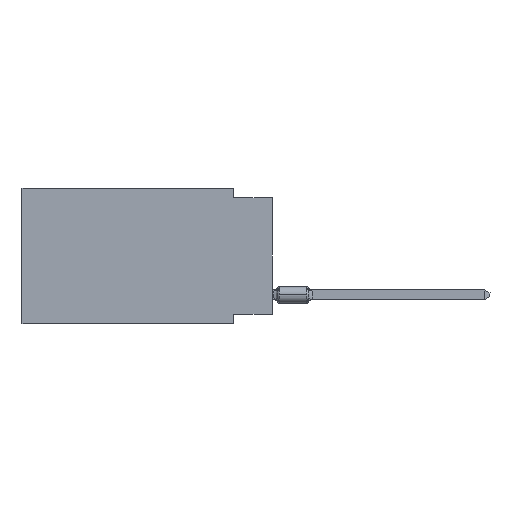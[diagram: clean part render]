
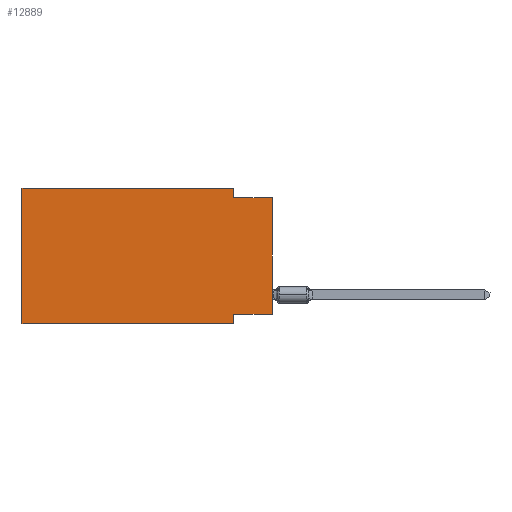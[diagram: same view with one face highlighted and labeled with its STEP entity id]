
A CAD part, left-side view. The second image highlights one B-rep face of the part: STEP entity #12889.
In plain terms, the highlighted planar face has unit normal (-1, 0, 0).
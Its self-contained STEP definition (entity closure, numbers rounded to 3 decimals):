
#615 = LINE ( 'NONE', #16042, #12600 ) ;
#970 = EDGE_CURVE ( 'NONE', #9840, #2239, #18600, .T. ) ;
#1143 = EDGE_CURVE ( 'NONE', #9840, #15726, #25029, .T. ) ;
#1150 = DIRECTION ( 'NONE',  ( 0., 0., -1. ) ) ;
#1346 = CARTESIAN_POINT ( 'NONE',  ( 0., 0., 0. ) ) ;
#1924 = CARTESIAN_POINT ( 'NONE',  ( 0., 16.383, -8.89 ) ) ;
#1976 = DIRECTION ( 'NONE',  ( 0., -1., 0. ) ) ;
#2064 = ORIENTED_EDGE ( 'NONE', *, *, #970, .F. ) ;
#2103 = LINE ( 'NONE', #22062, #3014 ) ;
#2239 = VERTEX_POINT ( 'NONE', #5810 ) ;
#2859 = VERTEX_POINT ( 'NONE', #17123 ) ;
#3014 = VECTOR ( 'NONE', #1976, 1000. ) ;
#3246 = ORIENTED_EDGE ( 'NONE', *, *, #18876, .F. ) ;
#3462 = EDGE_LOOP ( 'NONE', ( #14455, #17822, #12158, #16643, #3246, #7448, #14622, #2064 ) ) ;
#3702 = LINE ( 'NONE', #7567, #4175 ) ;
#4145 = FACE_OUTER_BOUND ( 'NONE', #3462, .T. ) ;
#4175 = VECTOR ( 'NONE', #11543, 1000. ) ;
#4711 = EDGE_CURVE ( 'NONE', #2239, #5932, #615, .T. ) ;
#4917 = EDGE_CURVE ( 'NONE', #11958, #22137, #24407, .T. ) ;
#5617 = CARTESIAN_POINT ( 'NONE',  ( 0., 16.383, 0. ) ) ;
#5810 = CARTESIAN_POINT ( 'NONE',  ( 0., 2.54, -8.255 ) ) ;
#5932 = VERTEX_POINT ( 'NONE', #16215 ) ;
#7036 = DIRECTION ( 'NONE',  ( 0., 0., -1. ) ) ;
#7448 = ORIENTED_EDGE ( 'NONE', *, *, #10541, .T. ) ;
#7567 = CARTESIAN_POINT ( 'NONE',  ( 0., 16.383, 0. ) ) ;
#8411 = VECTOR ( 'NONE', #8682, 1000. ) ;
#8682 = DIRECTION ( 'NONE',  ( 0., -1., 0. ) ) ;
#8826 = CARTESIAN_POINT ( 'NONE',  ( 0., 0., -8.255 ) ) ;
#9204 = DIRECTION ( 'NONE',  ( 0., 0., 1. ) ) ;
#9279 = DIRECTION ( 'NONE',  ( 0., -1., 0. ) ) ;
#9840 = VERTEX_POINT ( 'NONE', #21013 ) ;
#10541 = EDGE_CURVE ( 'NONE', #2859, #5932, #15173, .T. ) ;
#10889 = VECTOR ( 'NONE', #16668, 1000. ) ;
#11504 = EDGE_CURVE ( 'NONE', #22137, #15726, #2103, .T. ) ;
#11543 = DIRECTION ( 'NONE',  ( 0., 0., 1. ) ) ;
#11562 = CARTESIAN_POINT ( 'NONE',  ( 0., 0., -0.635 ) ) ;
#11958 = VERTEX_POINT ( 'NONE', #14538 ) ;
#12058 = CARTESIAN_POINT ( 'NONE',  ( 0., 2.54, -0.635 ) ) ;
#12158 = ORIENTED_EDGE ( 'NONE', *, *, #4917, .F. ) ;
#12600 = VECTOR ( 'NONE', #19667, 1000. ) ;
#12889 = ADVANCED_FACE ( 'NONE', ( #4145 ), #19583, .F. ) ;
#14253 = VECTOR ( 'NONE', #7036, 1000. ) ;
#14455 = ORIENTED_EDGE ( 'NONE', *, *, #1143, .T. ) ;
#14538 = CARTESIAN_POINT ( 'NONE',  ( 0., 2.54, 0. ) ) ;
#14582 = CARTESIAN_POINT ( 'NONE',  ( 0., 16.383, 0. ) ) ;
#14622 = ORIENTED_EDGE ( 'NONE', *, *, #4711, .F. ) ;
#15173 = LINE ( 'NONE', #1924, #21056 ) ;
#15726 = VERTEX_POINT ( 'NONE', #11562 ) ;
#16042 = CARTESIAN_POINT ( 'NONE',  ( 0., 2.54, -8.89 ) ) ;
#16215 = CARTESIAN_POINT ( 'NONE',  ( 0., 2.54, -8.89 ) ) ;
#16643 = ORIENTED_EDGE ( 'NONE', *, *, #21086, .F. ) ;
#16668 = DIRECTION ( 'NONE',  ( 0., 1., 0. ) ) ;
#17057 = VECTOR ( 'NONE', #9204, 1000. ) ;
#17123 = CARTESIAN_POINT ( 'NONE',  ( 0., 16.383, -8.89 ) ) ;
#17822 = ORIENTED_EDGE ( 'NONE', *, *, #11504, .F. ) ;
#18600 = LINE ( 'NONE', #8826, #10889 ) ;
#18654 = DIRECTION ( 'NONE',  ( 1., 0., 0. ) ) ;
#18749 = CARTESIAN_POINT ( 'NONE',  ( 0., 2.54, 0. ) ) ;
#18876 = EDGE_CURVE ( 'NONE', #2859, #22403, #3702, .T. ) ;
#19583 = PLANE ( 'NONE',  #19713 ) ;
#19667 = DIRECTION ( 'NONE',  ( 0., 0., -1. ) ) ;
#19713 = AXIS2_PLACEMENT_3D ( 'NONE', #20586, #18654, #1150 ) ;
#20586 = CARTESIAN_POINT ( 'NONE',  ( 0., 16.383, 0. ) ) ;
#20889 = LINE ( 'NONE', #14582, #8411 ) ;
#21013 = CARTESIAN_POINT ( 'NONE',  ( 0., 0., -8.255 ) ) ;
#21056 = VECTOR ( 'NONE', #9279, 1000. ) ;
#21086 = EDGE_CURVE ( 'NONE', #22403, #11958, #20889, .T. ) ;
#22062 = CARTESIAN_POINT ( 'NONE',  ( 0., 0., -0.635 ) ) ;
#22137 = VERTEX_POINT ( 'NONE', #12058 ) ;
#22403 = VERTEX_POINT ( 'NONE', #5617 ) ;
#24407 = LINE ( 'NONE', #18749, #14253 ) ;
#25029 = LINE ( 'NONE', #1346, #17057 ) ;
